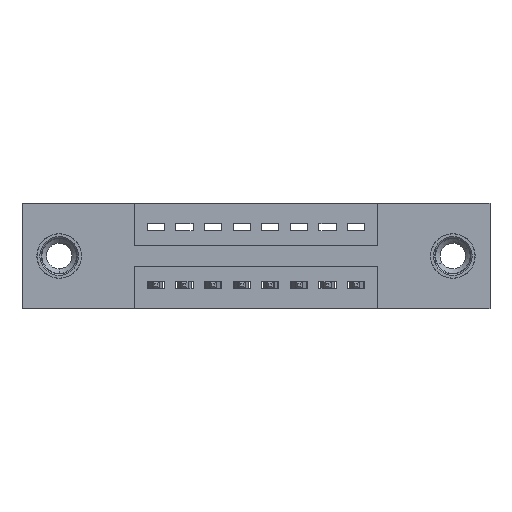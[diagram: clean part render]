
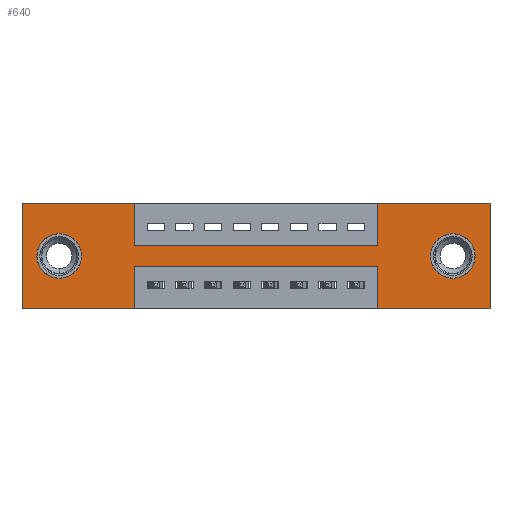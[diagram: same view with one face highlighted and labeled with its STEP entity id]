
A CAD part, front view. The second image highlights one B-rep face of the part: STEP entity #640.
In plain terms, the highlighted planar face has unit normal (0, -1, 0).
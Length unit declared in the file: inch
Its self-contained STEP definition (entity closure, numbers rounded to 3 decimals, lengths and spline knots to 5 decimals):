
#52 = LINE ( 'NONE', #6502, #7319 ) ;
#70 = VECTOR ( 'NONE', #3949, 39.37008 ) ;
#110 = AXIS2_PLACEMENT_3D ( 'NONE', #11690, #6514, #893 ) ;
#193 = EDGE_CURVE ( 'NONE', #8899, #5054, #11649, .T. ) ;
#221 = CARTESIAN_POINT ( 'NONE',  ( 0.3925, 0., -0.37 ) ) ;
#265 = DIRECTION ( 'NONE',  ( 0., 0., 1. ) ) ;
#493 = VERTEX_POINT ( 'NONE', #6942 ) ;
#570 = LINE ( 'NONE', #9662, #10296 ) ;
#594 = DIRECTION ( 'NONE',  ( 0., 0., 1. ) ) ;
#619 = ORIENTED_EDGE ( 'NONE', *, *, #8894, .F. ) ;
#640 = ADVANCED_FACE ( 'NONE', ( #5801, #9936, #7619 ), #10255, .T. ) ;
#743 = AXIS2_PLACEMENT_3D ( 'NONE', #11814, #10110, #10679 ) ;
#751 = ORIENTED_EDGE ( 'NONE', *, *, #5197, .F. ) ;
#830 = VECTOR ( 'NONE', #4390, 39.37008 ) ;
#882 = DIRECTION ( 'NONE',  ( -1., 0., 0. ) ) ;
#893 = DIRECTION ( 'NONE',  ( 0., 0., -1. ) ) ;
#997 = CARTESIAN_POINT ( 'NONE',  ( 0.3925, 0., -0.37 ) ) ;
#1236 = CARTESIAN_POINT ( 'NONE',  ( 1.2425, 0., -0.22 ) ) ;
#1241 = EDGE_CURVE ( 'NONE', #3020, #4028, #7963, .T. ) ;
#1707 = EDGE_LOOP ( 'NONE', ( #6208, #7915 ) ) ;
#1751 = CARTESIAN_POINT ( 'NONE',  ( 1.505, 0., -0.185 ) ) ;
#1823 = VECTOR ( 'NONE', #9444, 39.37008 ) ;
#1947 = VECTOR ( 'NONE', #5902, 39.37008 ) ;
#2092 = VERTEX_POINT ( 'NONE', #11074 ) ;
#2120 = LINE ( 'NONE', #221, #1823 ) ;
#2266 = EDGE_CURVE ( 'NONE', #11060, #10701, #5281, .T. ) ;
#2519 = VERTEX_POINT ( 'NONE', #6405 ) ;
#2534 = CARTESIAN_POINT ( 'NONE',  ( 0., 0., 0. ) ) ;
#2657 = ORIENTED_EDGE ( 'NONE', *, *, #5366, .F. ) ;
#2699 = DIRECTION ( 'NONE',  ( 0., 0., -1. ) ) ;
#2850 = DIRECTION ( 'NONE',  ( 0., 0., -1. ) ) ;
#3020 = VERTEX_POINT ( 'NONE', #6202 ) ;
#3098 = VERTEX_POINT ( 'NONE', #11471 ) ;
#3103 = CARTESIAN_POINT ( 'NONE',  ( 0., 0., 0. ) ) ;
#3137 = EDGE_CURVE ( 'NONE', #8781, #3098, #8203, .T. ) ;
#3790 = DIRECTION ( 'NONE',  ( -1., 0., 0. ) ) ;
#3890 = VECTOR ( 'NONE', #5247, 39.37008 ) ;
#3949 = DIRECTION ( 'NONE',  ( 1., 0., 0. ) ) ;
#4028 = VERTEX_POINT ( 'NONE', #9432 ) ;
#4041 = VERTEX_POINT ( 'NONE', #1236 ) ;
#4062 = CARTESIAN_POINT ( 'NONE',  ( 0., 0., -0.37 ) ) ;
#4203 = CARTESIAN_POINT ( 'NONE',  ( 1.2425, 0., -0.37 ) ) ;
#4207 = ORIENTED_EDGE ( 'NONE', *, *, #7015, .F. ) ;
#4241 = VERTEX_POINT ( 'NONE', #2534 ) ;
#4282 = EDGE_CURVE ( 'NONE', #9471, #3020, #7752, .T. ) ;
#4297 = CARTESIAN_POINT ( 'NONE',  ( 0.13, 0., -0.185 ) ) ;
#4313 = CARTESIAN_POINT ( 'NONE',  ( 0., 0., 0. ) ) ;
#4390 = DIRECTION ( 'NONE',  ( 1., 0., 0. ) ) ;
#4423 = LINE ( 'NONE', #4062, #1947 ) ;
#4836 = AXIS2_PLACEMENT_3D ( 'NONE', #1751, #8154, #2699 ) ;
#5054 = VERTEX_POINT ( 'NONE', #11722 ) ;
#5147 = DIRECTION ( 'NONE',  ( 0., 0., -1. ) ) ;
#5168 = VERTEX_POINT ( 'NONE', #7610 ) ;
#5197 = EDGE_CURVE ( 'NONE', #4241, #11060, #5218, .T. ) ;
#5218 = LINE ( 'NONE', #3103, #70 ) ;
#5229 = DIRECTION ( 'NONE',  ( 0., 0., 1. ) ) ;
#5247 = DIRECTION ( 'NONE',  ( 0., 0., 1. ) ) ;
#5281 = LINE ( 'NONE', #11261, #5576 ) ;
#5296 = EDGE_CURVE ( 'NONE', #2519, #4041, #10837, .T. ) ;
#5366 = EDGE_CURVE ( 'NONE', #10701, #9471, #570, .T. ) ;
#5505 = VECTOR ( 'NONE', #3790, 39.37008 ) ;
#5576 = VECTOR ( 'NONE', #5147, 39.37008 ) ;
#5627 = EDGE_CURVE ( 'NONE', #4028, #5168, #52, .T. ) ;
#5686 = AXIS2_PLACEMENT_3D ( 'NONE', #9248, #9236, #9235 ) ;
#5782 = VECTOR ( 'NONE', #882, 39.37008 ) ;
#5801 = FACE_BOUND ( 'NONE', #1707, .T. ) ;
#5902 = DIRECTION ( 'NONE',  ( -1., 0., 0. ) ) ;
#6051 = LINE ( 'NONE', #11682, #5782 ) ;
#6149 = DIRECTION ( 'NONE',  ( 1., 0., 0. ) ) ;
#6202 = CARTESIAN_POINT ( 'NONE',  ( 1.2425, 0., 0. ) ) ;
#6208 = ORIENTED_EDGE ( 'NONE', *, *, #11068, .T. ) ;
#6351 = CARTESIAN_POINT ( 'NONE',  ( 1.505, 0., -0.263 ) ) ;
#6405 = CARTESIAN_POINT ( 'NONE',  ( 1.2425, 0., -0.37 ) ) ;
#6471 = CARTESIAN_POINT ( 'NONE',  ( 0.3925, 0., 0. ) ) ;
#6502 = CARTESIAN_POINT ( 'NONE',  ( 1.635, 0., 0. ) ) ;
#6514 = DIRECTION ( 'NONE',  ( 0., 1., 0. ) ) ;
#6637 = CIRCLE ( 'NONE', #6685, 0.078 ) ;
#6685 = AXIS2_PLACEMENT_3D ( 'NONE', #4297, #10476, #5229 ) ;
#6942 = CARTESIAN_POINT ( 'NONE',  ( 0.3925, 0., -0.22 ) ) ;
#7015 = EDGE_CURVE ( 'NONE', #493, #9595, #2120, .T. ) ;
#7079 = ORIENTED_EDGE ( 'NONE', *, *, #1241, .F. ) ;
#7207 = ORIENTED_EDGE ( 'NONE', *, *, #7969, .T. ) ;
#7319 = VECTOR ( 'NONE', #2850, 39.37008 ) ;
#7365 = ORIENTED_EDGE ( 'NONE', *, *, #193, .T. ) ;
#7449 = CARTESIAN_POINT ( 'NONE',  ( 0.13, 0., -0.263 ) ) ;
#7466 = EDGE_LOOP ( 'NONE', ( #7207, #7365 ) ) ;
#7610 = CARTESIAN_POINT ( 'NONE',  ( 1.635, 0., -0.37 ) ) ;
#7619 = FACE_OUTER_BOUND ( 'NONE', #7808, .T. ) ;
#7752 = LINE ( 'NONE', #11451, #9799 ) ;
#7808 = EDGE_LOOP ( 'NONE', ( #4207, #10093, #9036, #9308, #11418, #7079, #11643, #2657, #9110, #751, #11796, #619 ) ) ;
#7915 = ORIENTED_EDGE ( 'NONE', *, *, #3137, .T. ) ;
#7963 = LINE ( 'NONE', #4313, #830 ) ;
#7969 = EDGE_CURVE ( 'NONE', #5054, #8899, #6637, .T. ) ;
#8154 = DIRECTION ( 'NONE',  ( 0., 1., 0. ) ) ;
#8203 = CIRCLE ( 'NONE', #4836, 0.078 ) ;
#8217 = CARTESIAN_POINT ( 'NONE',  ( 1.2425, 0., -0.15 ) ) ;
#8565 = VECTOR ( 'NONE', #265, 39.37008 ) ;
#8657 = CIRCLE ( 'NONE', #110, 0.078 ) ;
#8781 = VERTEX_POINT ( 'NONE', #6351 ) ;
#8878 = EDGE_CURVE ( 'NONE', #4041, #493, #6051, .T. ) ;
#8894 = EDGE_CURVE ( 'NONE', #9595, #2092, #10165, .T. ) ;
#8899 = VERTEX_POINT ( 'NONE', #7449 ) ;
#8973 = LINE ( 'NONE', #9653, #3890 ) ;
#9036 = ORIENTED_EDGE ( 'NONE', *, *, #5296, .F. ) ;
#9110 = ORIENTED_EDGE ( 'NONE', *, *, #2266, .F. ) ;
#9233 = EDGE_CURVE ( 'NONE', #2092, #4241, #8973, .T. ) ;
#9235 = DIRECTION ( 'NONE',  ( 0., 0., 1. ) ) ;
#9236 = DIRECTION ( 'NONE',  ( 0., 1., 0. ) ) ;
#9248 = CARTESIAN_POINT ( 'NONE',  ( 0.13, 0., -0.185 ) ) ;
#9308 = ORIENTED_EDGE ( 'NONE', *, *, #11804, .F. ) ;
#9348 = CARTESIAN_POINT ( 'NONE',  ( 0.3925, 0., -0.15 ) ) ;
#9432 = CARTESIAN_POINT ( 'NONE',  ( 1.635, 0., 0. ) ) ;
#9444 = DIRECTION ( 'NONE',  ( 0., 0., -1. ) ) ;
#9471 = VERTEX_POINT ( 'NONE', #8217 ) ;
#9595 = VERTEX_POINT ( 'NONE', #997 ) ;
#9653 = CARTESIAN_POINT ( 'NONE',  ( 0., 0., 0. ) ) ;
#9662 = CARTESIAN_POINT ( 'NONE',  ( 0.3925, 0., -0.15 ) ) ;
#9799 = VECTOR ( 'NONE', #594, 39.37008 ) ;
#9936 = FACE_BOUND ( 'NONE', #7466, .T. ) ;
#10033 = CARTESIAN_POINT ( 'NONE',  ( 0., 0., -0.37 ) ) ;
#10093 = ORIENTED_EDGE ( 'NONE', *, *, #8878, .F. ) ;
#10110 = DIRECTION ( 'NONE',  ( 0., -1., 0. ) ) ;
#10165 = LINE ( 'NONE', #10033, #5505 ) ;
#10255 = PLANE ( 'NONE',  #743 ) ;
#10296 = VECTOR ( 'NONE', #6149, 39.37008 ) ;
#10476 = DIRECTION ( 'NONE',  ( 0., 1., 0. ) ) ;
#10679 = DIRECTION ( 'NONE',  ( 0., 0., -1. ) ) ;
#10701 = VERTEX_POINT ( 'NONE', #9348 ) ;
#10837 = LINE ( 'NONE', #4203, #8565 ) ;
#11060 = VERTEX_POINT ( 'NONE', #6471 ) ;
#11068 = EDGE_CURVE ( 'NONE', #3098, #8781, #8657, .T. ) ;
#11074 = CARTESIAN_POINT ( 'NONE',  ( 0., 0., -0.37 ) ) ;
#11261 = CARTESIAN_POINT ( 'NONE',  ( 0.3925, 0., 0. ) ) ;
#11418 = ORIENTED_EDGE ( 'NONE', *, *, #5627, .F. ) ;
#11451 = CARTESIAN_POINT ( 'NONE',  ( 1.2425, 0., 0. ) ) ;
#11471 = CARTESIAN_POINT ( 'NONE',  ( 1.505, 0., -0.107 ) ) ;
#11643 = ORIENTED_EDGE ( 'NONE', *, *, #4282, .F. ) ;
#11649 = CIRCLE ( 'NONE', #5686, 0.078 ) ;
#11682 = CARTESIAN_POINT ( 'NONE',  ( 0.3925, 0., -0.22 ) ) ;
#11690 = CARTESIAN_POINT ( 'NONE',  ( 1.505, 0., -0.185 ) ) ;
#11722 = CARTESIAN_POINT ( 'NONE',  ( 0.13, 0., -0.107 ) ) ;
#11796 = ORIENTED_EDGE ( 'NONE', *, *, #9233, .F. ) ;
#11804 = EDGE_CURVE ( 'NONE', #5168, #2519, #4423, .T. ) ;
#11814 = CARTESIAN_POINT ( 'NONE',  ( 0., 0., -0.37 ) ) ;
